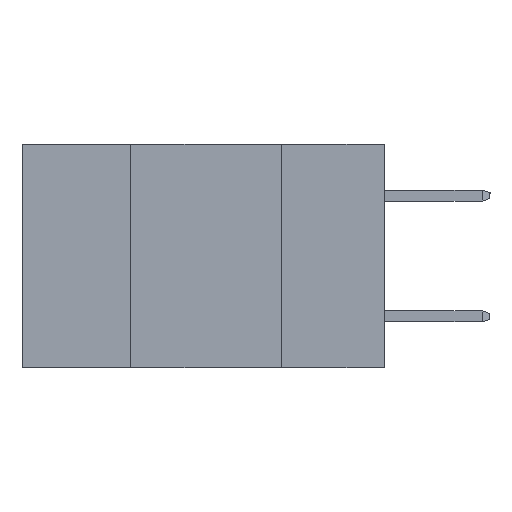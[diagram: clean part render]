
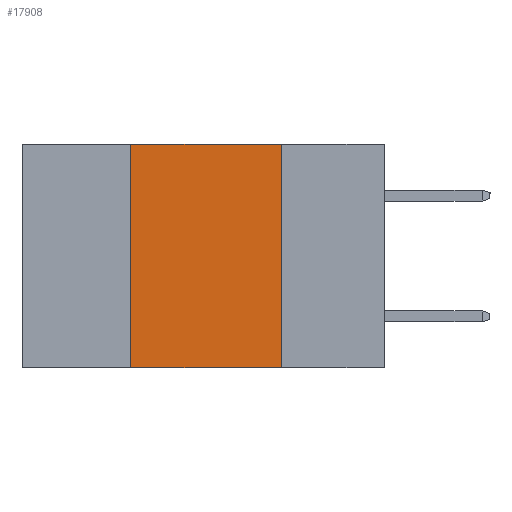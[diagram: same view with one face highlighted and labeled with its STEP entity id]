
A CAD part, left-side view. The second image highlights one B-rep face of the part: STEP entity #17908.
In plain terms, the highlighted planar face has unit normal (-1, 0, 0).
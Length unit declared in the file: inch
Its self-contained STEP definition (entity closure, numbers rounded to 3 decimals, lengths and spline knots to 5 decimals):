
#250 = AXIS2_PLACEMENT_3D ( 'NONE', #3519, #15599, #23444 ) ;
#753 = ORIENTED_EDGE ( 'NONE', *, *, #24306, .F. ) ;
#1324 = DIRECTION ( 'NONE',  ( 0., 0., 1. ) ) ;
#1574 = CARTESIAN_POINT ( 'NONE',  ( 0., 0.42, -0.37 ) ) ;
#2207 = ORIENTED_EDGE ( 'NONE', *, *, #19426, .F. ) ;
#3519 = CARTESIAN_POINT ( 'NONE',  ( 0., 0.6, 0. ) ) ;
#3941 = ORIENTED_EDGE ( 'NONE', *, *, #6140, .T. ) ;
#4387 = VERTEX_POINT ( 'NONE', #20179 ) ;
#5650 = ORIENTED_EDGE ( 'NONE', *, *, #7039, .F. ) ;
#5925 = CARTESIAN_POINT ( 'NONE',  ( 0., 0.42, -0.37 ) ) ;
#6026 = VECTOR ( 'NONE', #15760, 39.37008 ) ;
#6140 = EDGE_CURVE ( 'NONE', #18760, #11554, #20600, .T. ) ;
#7039 = EDGE_CURVE ( 'NONE', #4387, #10942, #21393, .T. ) ;
#8478 = VECTOR ( 'NONE', #1324, 39.37008 ) ;
#9684 = FACE_OUTER_BOUND ( 'NONE', #24200, .T. ) ;
#9721 = LINE ( 'NONE', #19737, #6026 ) ;
#10942 = VERTEX_POINT ( 'NONE', #11495 ) ;
#10975 = DIRECTION ( 'NONE',  ( 0., -1., 0. ) ) ;
#11495 = CARTESIAN_POINT ( 'NONE',  ( 0., 0.17, 0. ) ) ;
#11554 = VERTEX_POINT ( 'NONE', #12959 ) ;
#12959 = CARTESIAN_POINT ( 'NONE',  ( 0., 0.17, -0.37 ) ) ;
#13702 = CARTESIAN_POINT ( 'NONE',  ( 0., 0.6, 0. ) ) ;
#14469 = VECTOR ( 'NONE', #23586, 39.37008 ) ;
#15474 = PLANE ( 'NONE',  #250 ) ;
#15599 = DIRECTION ( 'NONE',  ( 1., 0., 0. ) ) ;
#15760 = DIRECTION ( 'NONE',  ( 0., 0., -1. ) ) ;
#17908 = ADVANCED_FACE ( 'NONE', ( #9684 ), #15474, .F. ) ;
#18680 = CARTESIAN_POINT ( 'NONE',  ( 0., 0.6, -0.37 ) ) ;
#18760 = VERTEX_POINT ( 'NONE', #5925 ) ;
#19299 = LINE ( 'NONE', #1574, #8478 ) ;
#19426 = EDGE_CURVE ( 'NONE', #10942, #11554, #9721, .T. ) ;
#19737 = CARTESIAN_POINT ( 'NONE',  ( 0., 0.17, -0.37 ) ) ;
#20179 = CARTESIAN_POINT ( 'NONE',  ( 0., 0.42, 0. ) ) ;
#20600 = LINE ( 'NONE', #18680, #25214 ) ;
#21393 = LINE ( 'NONE', #13702, #14469 ) ;
#23444 = DIRECTION ( 'NONE',  ( 0., 0., -1. ) ) ;
#23586 = DIRECTION ( 'NONE',  ( 0., -1., 0. ) ) ;
#24200 = EDGE_LOOP ( 'NONE', ( #2207, #5650, #753, #3941 ) ) ;
#24306 = EDGE_CURVE ( 'NONE', #18760, #4387, #19299, .T. ) ;
#25214 = VECTOR ( 'NONE', #10975, 39.37008 ) ;
